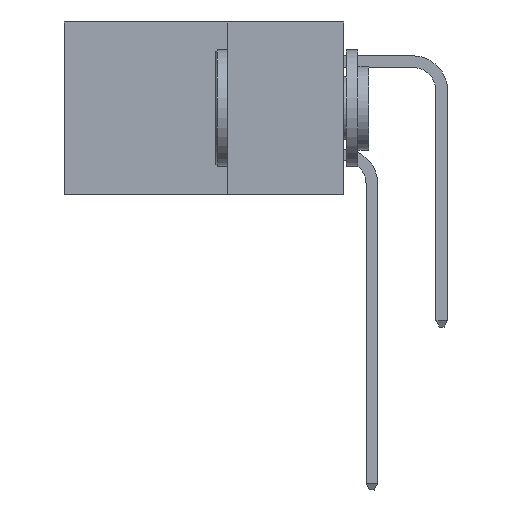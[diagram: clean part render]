
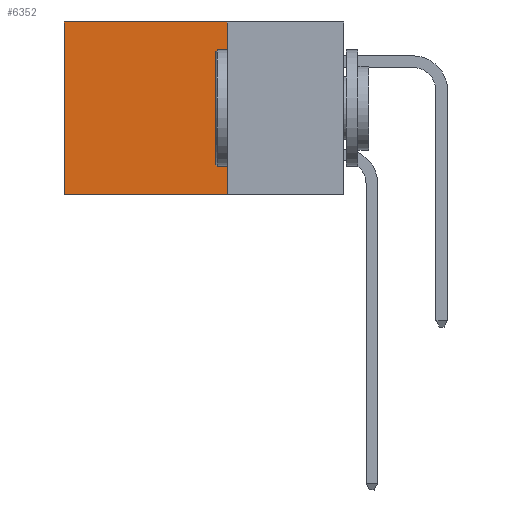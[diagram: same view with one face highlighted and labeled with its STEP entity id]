
A CAD part, left-side view. The second image highlights one B-rep face of the part: STEP entity #6352.
In plain terms, the highlighted planar face has unit normal (-1, 0, 0).
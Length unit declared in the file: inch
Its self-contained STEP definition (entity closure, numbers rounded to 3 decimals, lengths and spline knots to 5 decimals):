
#97 = AXIS2_PLACEMENT_3D ( 'NONE', #25664, #12991, #25285 ) ;
#764 = VECTOR ( 'NONE', #14994, 39.37008 ) ;
#1466 = LINE ( 'NONE', #27153, #764 ) ;
#3147 = VECTOR ( 'NONE', #8729, 39.37008 ) ;
#3167 = EDGE_CURVE ( 'NONE', #22009, #24708, #19146, .T. ) ;
#4029 = ORIENTED_EDGE ( 'NONE', *, *, #3167, .F. ) ;
#4139 = VERTEX_POINT ( 'NONE', #8101 ) ;
#5989 = DIRECTION ( 'NONE',  ( 0., 0., -1. ) ) ;
#6352 = ADVANCED_FACE ( 'NONE', ( #19940 ), #21503, .F. ) ;
#6570 = CARTESIAN_POINT ( 'NONE',  ( 0.298, 0.6, 0. ) ) ;
#7361 = CARTESIAN_POINT ( 'NONE',  ( 0.298, 0.25, -0.37 ) ) ;
#7843 = VECTOR ( 'NONE', #5989, 39.37008 ) ;
#8101 = CARTESIAN_POINT ( 'NONE',  ( 0.298, 0.6, -0.37 ) ) ;
#8406 = VERTEX_POINT ( 'NONE', #14148 ) ;
#8729 = DIRECTION ( 'NONE',  ( 0., 0., -1. ) ) ;
#8943 = LINE ( 'NONE', #6570, #3147 ) ;
#10055 = ORIENTED_EDGE ( 'NONE', *, *, #15580, .T. ) ;
#12321 = EDGE_CURVE ( 'NONE', #24708, #4139, #26389, .T. ) ;
#12991 = DIRECTION ( 'NONE',  ( 1., 0., 0. ) ) ;
#13258 = CARTESIAN_POINT ( 'NONE',  ( 0.298, 0.25, 0. ) ) ;
#13944 = CARTESIAN_POINT ( 'NONE',  ( 0.298, 0.25, 0. ) ) ;
#14148 = CARTESIAN_POINT ( 'NONE',  ( 0.298, 0.6, 0. ) ) ;
#14994 = DIRECTION ( 'NONE',  ( 0., 1., 0. ) ) ;
#15567 = ORIENTED_EDGE ( 'NONE', *, *, #12321, .F. ) ;
#15580 = EDGE_CURVE ( 'NONE', #22009, #8406, #1466, .T. ) ;
#16609 = DIRECTION ( 'NONE',  ( 0., 1., 0. ) ) ;
#17727 = EDGE_LOOP ( 'NONE', ( #25141, #15567, #4029, #10055 ) ) ;
#19146 = LINE ( 'NONE', #13944, #7843 ) ;
#19940 = FACE_OUTER_BOUND ( 'NONE', #17727, .T. ) ;
#21503 = PLANE ( 'NONE',  #97 ) ;
#22009 = VERTEX_POINT ( 'NONE', #13258 ) ;
#24686 = CARTESIAN_POINT ( 'NONE',  ( 0.298, 0.25, -0.37 ) ) ;
#24708 = VERTEX_POINT ( 'NONE', #7361 ) ;
#25141 = ORIENTED_EDGE ( 'NONE', *, *, #25802, .T. ) ;
#25285 = DIRECTION ( 'NONE',  ( 0., 0., -1. ) ) ;
#25664 = CARTESIAN_POINT ( 'NONE',  ( 0.298, 0.25, 0. ) ) ;
#25802 = EDGE_CURVE ( 'NONE', #8406, #4139, #8943, .T. ) ;
#26389 = LINE ( 'NONE', #24686, #27040 ) ;
#27040 = VECTOR ( 'NONE', #16609, 39.37008 ) ;
#27153 = CARTESIAN_POINT ( 'NONE',  ( 0.298, 0.25, 0. ) ) ;
